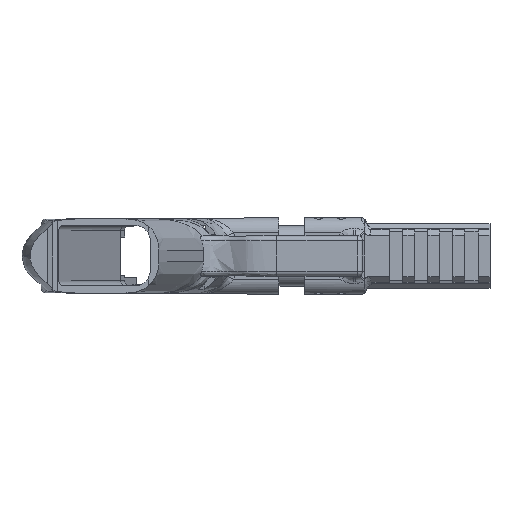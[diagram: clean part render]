
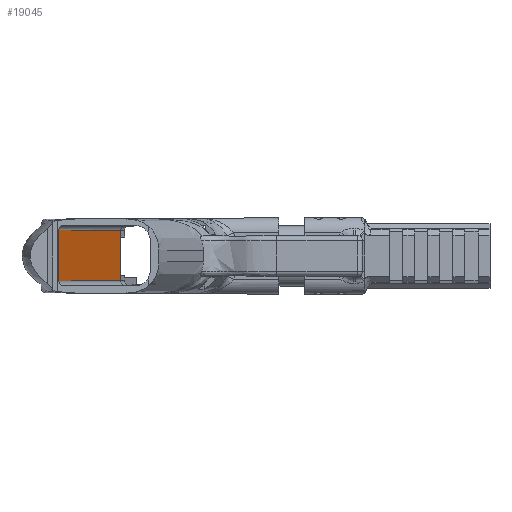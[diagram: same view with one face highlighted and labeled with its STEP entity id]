
A CAD part, front view. The second image highlights one B-rep face of the part: STEP entity #19045.
In plain terms, the highlighted planar face has unit normal (0.956, -0.292, 0).
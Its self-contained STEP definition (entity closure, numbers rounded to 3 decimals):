
#4496 = VECTOR ( 'NONE', #58379, 1000. ) ;
#4677 = LINE ( 'NONE', #113599, #4496 ) ;
#4943 = CARTESIAN_POINT ( 'NONE',  ( 38.813, 16.845, -25.15 ) ) ;
#6135 = DIRECTION ( 'NONE',  ( 0.292, 0.956, 0. ) ) ;
#16333 = VECTOR ( 'NONE', #102930, 1000. ) ;
#19045 = ADVANCED_FACE ( 'NONE', ( #138290 ), #38779, .T. ) ;
#22780 = EDGE_CURVE ( 'NONE', #78077, #137723, #4677, .T. ) ;
#23598 = CARTESIAN_POINT ( 'NONE',  ( 6.978, -87.285, -25.15 ) ) ;
#24918 = VECTOR ( 'NONE', #122653, 1000. ) ;
#31168 = CARTESIAN_POINT ( 'NONE',  ( 31.554, -6.9, -131.166 ) ) ;
#37159 = VECTOR ( 'NONE', #92349, 1000. ) ;
#38779 = PLANE ( 'NONE',  #143549 ) ;
#40966 = ORIENTED_EDGE ( 'NONE', *, *, #22780, .F. ) ;
#51920 = ORIENTED_EDGE ( 'NONE', *, *, #110786, .F. ) ;
#58379 = DIRECTION ( 'NONE',  ( 0., 0., 1. ) ) ;
#61271 = CARTESIAN_POINT ( 'NONE',  ( 38.813, 16.845, -131.166 ) ) ;
#62911 = CARTESIAN_POINT ( 'NONE',  ( 31.554, -6.9, -25.15 ) ) ;
#64923 = EDGE_CURVE ( 'NONE', #111980, #137723, #112700, .T. ) ;
#71183 = CARTESIAN_POINT ( 'NONE',  ( 31.554, -6.9, -5. ) ) ;
#78077 = VERTEX_POINT ( 'NONE', #23598 ) ;
#85071 = CARTESIAN_POINT ( 'NONE',  ( 6.978, -87.285, -5. ) ) ;
#92349 = DIRECTION ( 'NONE',  ( -0.292, -0.956, 0. ) ) ;
#100116 = LINE ( 'NONE', #31168, #24918 ) ;
#102930 = DIRECTION ( 'NONE',  ( -0.292, -0.956, 0. ) ) ;
#103229 = CARTESIAN_POINT ( 'NONE',  ( 38.813, 16.845, -5. ) ) ;
#105585 = DIRECTION ( 'NONE',  ( 0.956, -0.292, 0. ) ) ;
#106759 = ORIENTED_EDGE ( 'NONE', *, *, #133390, .F. ) ;
#107843 = ORIENTED_EDGE ( 'NONE', *, *, #64923, .T. ) ;
#110786 = EDGE_CURVE ( 'NONE', #119015, #78077, #137789, .T. ) ;
#111980 = VERTEX_POINT ( 'NONE', #71183 ) ;
#112700 = LINE ( 'NONE', #103229, #37159 ) ;
#113599 = CARTESIAN_POINT ( 'NONE',  ( 6.978, -87.285, -131.166 ) ) ;
#118448 = EDGE_LOOP ( 'NONE', ( #106759, #107843, #40966, #51920 ) ) ;
#119015 = VERTEX_POINT ( 'NONE', #62911 ) ;
#122653 = DIRECTION ( 'NONE',  ( 0., 0., -1. ) ) ;
#133390 = EDGE_CURVE ( 'NONE', #111980, #119015, #100116, .T. ) ;
#137723 = VERTEX_POINT ( 'NONE', #85071 ) ;
#137789 = LINE ( 'NONE', #4943, #16333 ) ;
#138290 = FACE_OUTER_BOUND ( 'NONE', #118448, .T. ) ;
#143549 = AXIS2_PLACEMENT_3D ( 'NONE', #61271, #105585, #6135 ) ;
